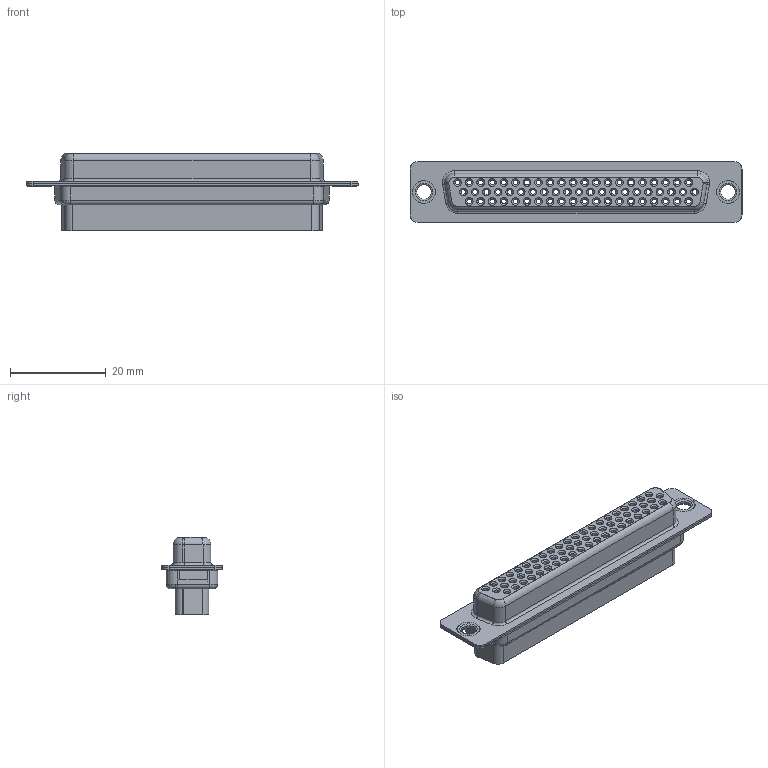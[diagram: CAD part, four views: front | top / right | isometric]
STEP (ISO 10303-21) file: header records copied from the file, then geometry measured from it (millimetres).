
FILE_DESCRIPTION (( 'STEP AP203' ), '1' );
FILE_NAME ('638-062-010-041.STEP', '2020-07-18T16:45:15', ( '' ), ( '' ), 'SwSTEP 2.0', 'SolidWorks 2020', '' );
FILE_SCHEMA (( 'CONFIG_CONTROL_DESIGN' ));
Length unit declared in the file: millimetre
Products named in the file (5): 638-062-010-041; 638 Thru Hole Rivet; 638 Housing_62 Contacts HP; 638 Shell Front_62 Contacts; 638 Shell Rear_62 Contacts
Assembly tree (5 placements, depth 2):
  638-062-010-041
    638 Housing_62 Contacts HP
    638 Shell Front_62 Contacts
    638 Shell Rear_62 Contacts
    638 Thru Hole Rivet  x2
Bounding box: 69.32 x 12.6 x 16.1 mm (x, y, z)
Volume: 4851.7 mm3; surface area: 12784 mm2
Topology: 5 solids, 5 shells, 1059 faces, 2339 edges, 1487 vertices
Faces by surface type: cylinder 617, plane 253, cone 124, torus 65
Entity records: 30065 total; most frequent: DIRECTION 5747, CARTESIAN_POINT 4993, ORIENTED_EDGE 4598, AXIS2_PLACEMENT_3D 2446, EDGE_CURVE 2299, VERTEX_POINT 1463, CIRCLE 1399, EDGE_LOOP 1372
